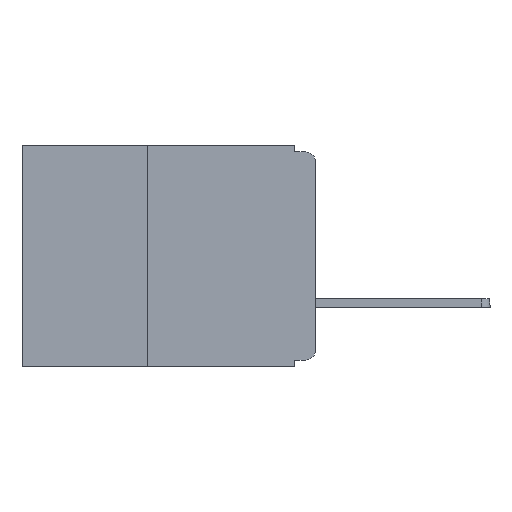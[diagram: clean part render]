
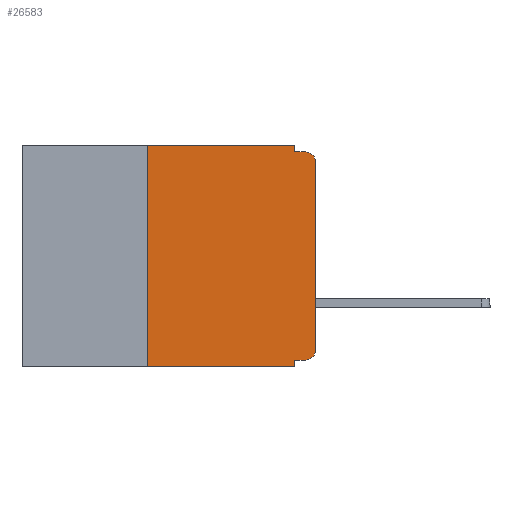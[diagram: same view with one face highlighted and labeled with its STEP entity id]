
A CAD part, left-side view. The second image highlights one B-rep face of the part: STEP entity #26583.
In plain terms, the highlighted planar face has unit normal (-1, 0, 0).
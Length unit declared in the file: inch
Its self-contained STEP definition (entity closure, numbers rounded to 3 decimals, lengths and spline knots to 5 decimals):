
#206 = VERTEX_POINT ( 'NONE', #15232 ) ;
#350 = VECTOR ( 'NONE', #1489, 39.37008 ) ;
#493 = AXIS2_PLACEMENT_3D ( 'NONE', #8863, #8855, #8826 ) ;
#901 = VECTOR ( 'NONE', #27318, 39.37008 ) ;
#975 = ORIENTED_EDGE ( 'NONE', *, *, #18792, .T. ) ;
#1051 = CARTESIAN_POINT ( 'NONE',  ( 0., 0.437, 0. ) ) ;
#1163 = VERTEX_POINT ( 'NONE', #21987 ) ;
#1489 = DIRECTION ( 'NONE',  ( 0., -1., 0. ) ) ;
#1792 = EDGE_CURVE ( 'NONE', #26563, #1163, #6649, .T. ) ;
#1815 = CARTESIAN_POINT ( 'NONE',  ( 0., 0., -0.32 ) ) ;
#2750 = FACE_OUTER_BOUND ( 'NONE', #13864, .T. ) ;
#2897 = DIRECTION ( 'NONE',  ( 0., 0., 1. ) ) ;
#2900 = EDGE_CURVE ( 'NONE', #12612, #11869, #21113, .T. ) ;
#3344 = VECTOR ( 'NONE', #4007, 39.37008 ) ;
#3594 = ORIENTED_EDGE ( 'NONE', *, *, #17845, .F. ) ;
#3740 = VECTOR ( 'NONE', #2897, 39.37008 ) ;
#3824 = CIRCLE ( 'NONE', #9484, 0.015 ) ;
#3872 = CARTESIAN_POINT ( 'NONE',  ( 0., 0.031, -0.33 ) ) ;
#3883 = VERTEX_POINT ( 'NONE', #18727 ) ;
#4007 = DIRECTION ( 'NONE',  ( 0., 1., 0. ) ) ;
#4025 = LINE ( 'NONE', #1815, #3344 ) ;
#4568 = VERTEX_POINT ( 'NONE', #8198 ) ;
#6649 = LINE ( 'NONE', #27218, #901 ) ;
#6763 = LINE ( 'NONE', #14295, #350 ) ;
#6971 = ORIENTED_EDGE ( 'NONE', *, *, #16953, .F. ) ;
#7124 = CARTESIAN_POINT ( 'NONE',  ( 0., 0.25, -0.33 ) ) ;
#7582 = LINE ( 'NONE', #21536, #12608 ) ;
#7776 = AXIS2_PLACEMENT_3D ( 'NONE', #15903, #11748, #26634 ) ;
#7820 = VECTOR ( 'NONE', #27340, 39.37008 ) ;
#8198 = CARTESIAN_POINT ( 'NONE',  ( 0., 0.25, -0.33 ) ) ;
#8233 = ORIENTED_EDGE ( 'NONE', *, *, #1792, .F. ) ;
#8826 = DIRECTION ( 'NONE',  ( 0., 0., -1. ) ) ;
#8855 = DIRECTION ( 'NONE',  ( -1., 0., 0. ) ) ;
#8863 = CARTESIAN_POINT ( 'NONE',  ( 0., 0.015, -0.025 ) ) ;
#9428 = EDGE_CURVE ( 'NONE', #206, #24347, #19128, .T. ) ;
#9484 = AXIS2_PLACEMENT_3D ( 'NONE', #11284, #26177, #13426 ) ;
#9682 = DIRECTION ( 'NONE',  ( 0., -1., 0. ) ) ;
#10065 = LINE ( 'NONE', #7124, #3740 ) ;
#10303 = LINE ( 'NONE', #1051, #14623 ) ;
#11171 = EDGE_CURVE ( 'NONE', #4568, #24347, #6763, .T. ) ;
#11284 = CARTESIAN_POINT ( 'NONE',  ( 0., 0.015, -0.305 ) ) ;
#11522 = EDGE_CURVE ( 'NONE', #4568, #23938, #10065, .T. ) ;
#11748 = DIRECTION ( 'NONE',  ( 1., 0., 0. ) ) ;
#11869 = VERTEX_POINT ( 'NONE', #21039 ) ;
#12464 = CARTESIAN_POINT ( 'NONE',  ( 0., 0., -0.01 ) ) ;
#12608 = VECTOR ( 'NONE', #23683, 39.37008 ) ;
#12612 = VERTEX_POINT ( 'NONE', #14440 ) ;
#13426 = DIRECTION ( 'NONE',  ( 0., 0., -1. ) ) ;
#13864 = EDGE_LOOP ( 'NONE', ( #975, #15720, #27359, #8233, #3594, #17769, #18470, #23892, #6971, #24987 ) ) ;
#14241 = VERTEX_POINT ( 'NONE', #26654 ) ;
#14295 = CARTESIAN_POINT ( 'NONE',  ( 0., 0.437, -0.33 ) ) ;
#14440 = CARTESIAN_POINT ( 'NONE',  ( 0., 0., -0.025 ) ) ;
#14564 = DIRECTION ( 'NONE',  ( 0., -1., 0. ) ) ;
#14623 = VECTOR ( 'NONE', #9682, 39.37008 ) ;
#15232 = CARTESIAN_POINT ( 'NONE',  ( 0., 0.031, -0.32 ) ) ;
#15720 = ORIENTED_EDGE ( 'NONE', *, *, #2900, .T. ) ;
#15735 = LINE ( 'NONE', #12464, #26432 ) ;
#15903 = CARTESIAN_POINT ( 'NONE',  ( 0., 0.437, 0. ) ) ;
#16706 = CARTESIAN_POINT ( 'NONE',  ( 0., 0.031, -0.33 ) ) ;
#16953 = EDGE_CURVE ( 'NONE', #14241, #206, #4025, .T. ) ;
#17769 = ORIENTED_EDGE ( 'NONE', *, *, #11522, .F. ) ;
#17845 = EDGE_CURVE ( 'NONE', #23938, #26563, #10303, .T. ) ;
#18470 = ORIENTED_EDGE ( 'NONE', *, *, #11171, .T. ) ;
#18727 = CARTESIAN_POINT ( 'NONE',  ( 0., 0., -0.305 ) ) ;
#18792 = EDGE_CURVE ( 'NONE', #3883, #12612, #7582, .T. ) ;
#19128 = LINE ( 'NONE', #3872, #7820 ) ;
#19695 = CARTESIAN_POINT ( 'NONE',  ( 0., 0.25, 0. ) ) ;
#21039 = CARTESIAN_POINT ( 'NONE',  ( 0., 0.015, -0.01 ) ) ;
#21113 = CIRCLE ( 'NONE', #493, 0.015 ) ;
#21536 = CARTESIAN_POINT ( 'NONE',  ( 0., 0., 0. ) ) ;
#21987 = CARTESIAN_POINT ( 'NONE',  ( 0., 0.031, -0.01 ) ) ;
#22352 = PLANE ( 'NONE',  #7776 ) ;
#22574 = EDGE_CURVE ( 'NONE', #14241, #3883, #3824, .T. ) ;
#23683 = DIRECTION ( 'NONE',  ( 0., 0., 1. ) ) ;
#23892 = ORIENTED_EDGE ( 'NONE', *, *, #9428, .F. ) ;
#23938 = VERTEX_POINT ( 'NONE', #19695 ) ;
#24347 = VERTEX_POINT ( 'NONE', #16706 ) ;
#24987 = ORIENTED_EDGE ( 'NONE', *, *, #22574, .T. ) ;
#26177 = DIRECTION ( 'NONE',  ( -1., 0., 0. ) ) ;
#26432 = VECTOR ( 'NONE', #14564, 39.37008 ) ;
#26541 = CARTESIAN_POINT ( 'NONE',  ( 0., 0.031, 0. ) ) ;
#26563 = VERTEX_POINT ( 'NONE', #26541 ) ;
#26583 = ADVANCED_FACE ( 'NONE', ( #2750 ), #22352, .F. ) ;
#26634 = DIRECTION ( 'NONE',  ( 0., 0., -1. ) ) ;
#26654 = CARTESIAN_POINT ( 'NONE',  ( 0., 0.015, -0.32 ) ) ;
#27218 = CARTESIAN_POINT ( 'NONE',  ( 0., 0.031, 0. ) ) ;
#27318 = DIRECTION ( 'NONE',  ( 0., 0., -1. ) ) ;
#27340 = DIRECTION ( 'NONE',  ( 0., 0., -1. ) ) ;
#27359 = ORIENTED_EDGE ( 'NONE', *, *, #27371, .F. ) ;
#27371 = EDGE_CURVE ( 'NONE', #1163, #11869, #15735, .T. ) ;
